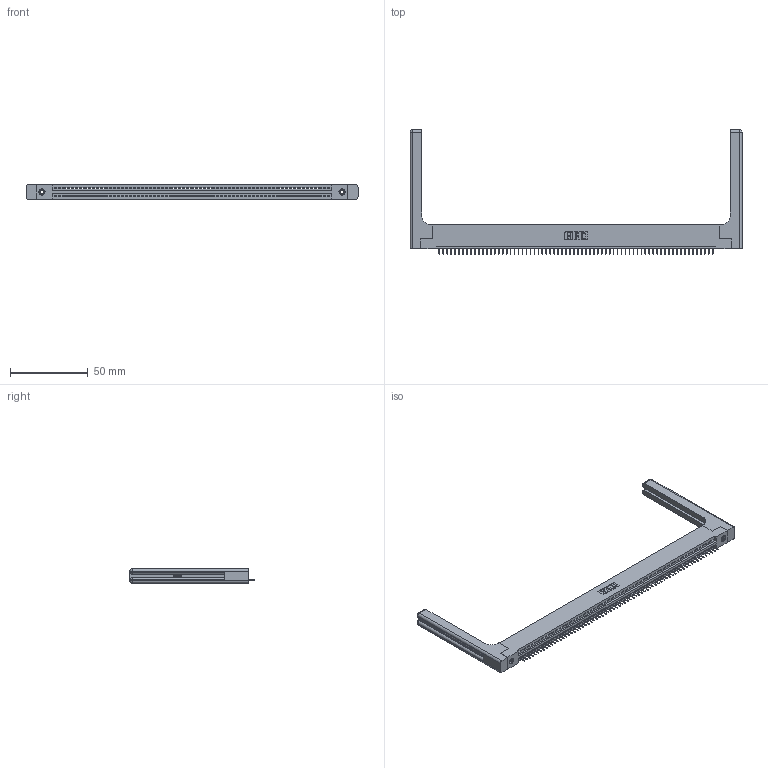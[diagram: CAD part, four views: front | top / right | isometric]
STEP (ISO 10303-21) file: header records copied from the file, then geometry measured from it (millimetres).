
FILE_DESCRIPTION (( 'STEP AP203' ), '1' );
FILE_NAME ('395-070-525-158.STEP', '2020-09-25T05:07:37', ( '' ), ( '' ), 'SwSTEP 2.0', 'SolidWorks 2020', '' );
FILE_SCHEMA (( 'CONFIG_CONTROL_DESIGN' ));
Length unit declared in the file: inch
Products named in the file (5): 345-292-001_345-293-125; 395-070-525-158; 345-250-001_345-250-001-102; 345-220-058_345-220-058; 345 Part_Flush Mounting Lugs - 0.156 Dia-TH
Assembly tree (75 placements, depth 2):
  395-070-525-158
    345 Part_Flush Mounting Lugs - 0.156 Dia-TH
    345-292-001_345-293-125  x70
    345-250-001_345-250-001-102  x2
    345-220-058_345-220-058  x2
Bounding box: 212.83 x 79.68 x 9.4 mm (x, y, z)
Volume: 28663 mm3; surface area: 31521.3 mm2
Topology: 75 solids, 75 shells, 4722 faces, 13607 edges, 8770 vertices
Faces by surface type: plane 3448, cylinder 1214, bspline 36, cone 12, sphere 8, torus 4
Entity records: 54170 total; most frequent: CARTESIAN_POINT 10351, ORIENTED_EDGE 9152, DIRECTION 7948, EDGE_CURVE 4576, LINE 4076, VECTOR 4076, VERTEX_POINT 3038, AXIS2_PLACEMENT_3D 1936
